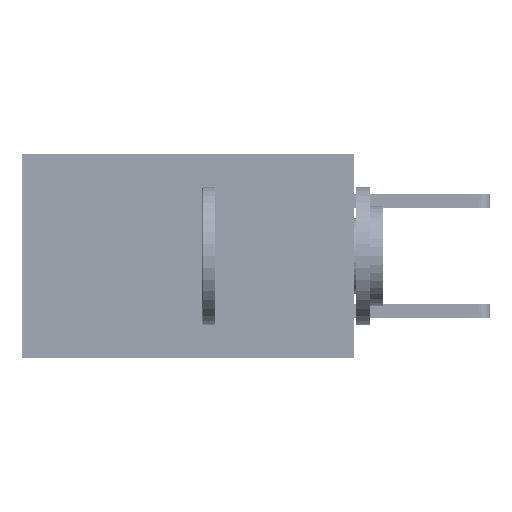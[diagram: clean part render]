
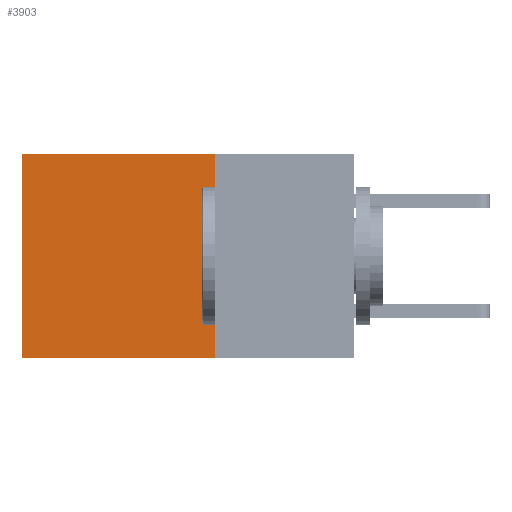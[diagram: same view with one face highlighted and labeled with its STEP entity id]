
A CAD part, left-side view. The second image highlights one B-rep face of the part: STEP entity #3903.
In plain terms, the highlighted planar face has unit normal (-1, 0, 0).
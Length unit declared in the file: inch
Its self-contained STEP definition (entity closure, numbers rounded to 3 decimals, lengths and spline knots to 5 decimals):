
#426 = CARTESIAN_POINT ( 'NONE',  ( 0.2875, 0.25, -0.37 ) ) ;
#2021 = ORIENTED_EDGE ( 'NONE', *, *, #40576, .T. ) ;
#2484 = CARTESIAN_POINT ( 'NONE',  ( 0.2875, 0.6, 0. ) ) ;
#2933 = VERTEX_POINT ( 'NONE', #8800 ) ;
#3207 = FACE_OUTER_BOUND ( 'NONE', #17054, .T. ) ;
#3632 = CARTESIAN_POINT ( 'NONE',  ( 0.2875, 0.25, 0. ) ) ;
#3652 = EDGE_CURVE ( 'NONE', #2933, #41748, #35776, .T. ) ;
#3903 = ADVANCED_FACE ( 'NONE', ( #3207 ), #37428, .F. ) ;
#3910 = CARTESIAN_POINT ( 'NONE',  ( 0.2875, 0.25, 0. ) ) ;
#7043 = CARTESIAN_POINT ( 'NONE',  ( 0.2875, 0.25, 0. ) ) ;
#8477 = CARTESIAN_POINT ( 'NONE',  ( 0.2875, 0.6, 0. ) ) ;
#8499 = LINE ( 'NONE', #19563, #33849 ) ;
#8800 = CARTESIAN_POINT ( 'NONE',  ( 0.2875, 0.25, 0. ) ) ;
#9607 = EDGE_CURVE ( 'NONE', #20183, #37422, #25181, .T. ) ;
#10582 = VECTOR ( 'NONE', #14164, 39.37008 ) ;
#11624 = ORIENTED_EDGE ( 'NONE', *, *, #41747, .F. ) ;
#13432 = DIRECTION ( 'NONE',  ( 0., 0., -1. ) ) ;
#14164 = DIRECTION ( 'NONE',  ( 0., 1., 0. ) ) ;
#14989 = VECTOR ( 'NONE', #41493, 39.37008 ) ;
#17054 = EDGE_LOOP ( 'NONE', ( #17168, #11624, #23705, #2021 ) ) ;
#17168 = ORIENTED_EDGE ( 'NONE', *, *, #9607, .T. ) ;
#17965 = DIRECTION ( 'NONE',  ( 0., 0., -1. ) ) ;
#19216 = LINE ( 'NONE', #7043, #10582 ) ;
#19563 = CARTESIAN_POINT ( 'NONE',  ( 0.2875, 0.25, -0.37 ) ) ;
#20183 = VERTEX_POINT ( 'NONE', #8477 ) ;
#23705 = ORIENTED_EDGE ( 'NONE', *, *, #3652, .F. ) ;
#25181 = LINE ( 'NONE', #2484, #14989 ) ;
#29678 = DIRECTION ( 'NONE',  ( 0., 1., 0. ) ) ;
#29804 = AXIS2_PLACEMENT_3D ( 'NONE', #3910, #34019, #17965 ) ;
#32220 = VECTOR ( 'NONE', #13432, 39.37008 ) ;
#33025 = CARTESIAN_POINT ( 'NONE',  ( 0.2875, 0.6, -0.37 ) ) ;
#33849 = VECTOR ( 'NONE', #29678, 39.37008 ) ;
#34019 = DIRECTION ( 'NONE',  ( 1., 0., 0. ) ) ;
#35776 = LINE ( 'NONE', #3632, #32220 ) ;
#37422 = VERTEX_POINT ( 'NONE', #33025 ) ;
#37428 = PLANE ( 'NONE',  #29804 ) ;
#40576 = EDGE_CURVE ( 'NONE', #2933, #20183, #19216, .T. ) ;
#41493 = DIRECTION ( 'NONE',  ( 0., 0., -1. ) ) ;
#41747 = EDGE_CURVE ( 'NONE', #41748, #37422, #8499, .T. ) ;
#41748 = VERTEX_POINT ( 'NONE', #426 ) ;
